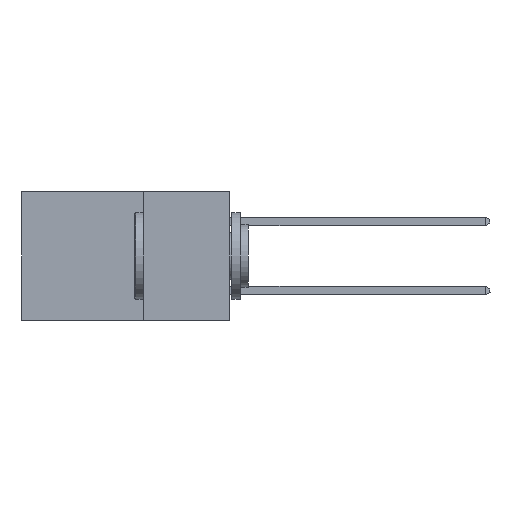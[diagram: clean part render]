
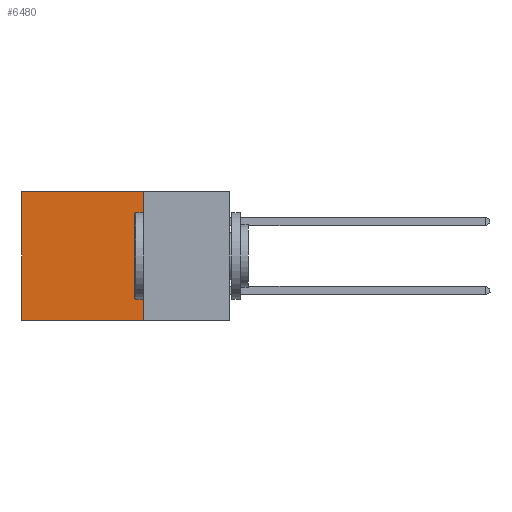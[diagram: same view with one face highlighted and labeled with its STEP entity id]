
A CAD part, left-side view. The second image highlights one B-rep face of the part: STEP entity #6480.
In plain terms, the highlighted planar face has unit normal (-1, 0, 0).
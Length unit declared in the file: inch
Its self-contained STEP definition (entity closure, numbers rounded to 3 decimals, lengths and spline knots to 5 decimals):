
#36 = FACE_OUTER_BOUND ( 'NONE', #13287, .T. ) ;
#1840 = LINE ( 'NONE', #17220, #14206 ) ;
#1922 = EDGE_CURVE ( 'NONE', #19029, #18520, #15356, .T. ) ;
#2025 = LINE ( 'NONE', #6024, #14391 ) ;
#2117 = CARTESIAN_POINT ( 'NONE',  ( 0.298, 0.25, -0.37 ) ) ;
#2572 = LINE ( 'NONE', #2117, #6442 ) ;
#2620 = ORIENTED_EDGE ( 'NONE', *, *, #1922, .T. ) ;
#6024 = CARTESIAN_POINT ( 'NONE',  ( 0.298, 0.25, 0. ) ) ;
#6319 = ORIENTED_EDGE ( 'NONE', *, *, #9165, .T. ) ;
#6348 = CARTESIAN_POINT ( 'NONE',  ( 0.298, 0.6, -0.37 ) ) ;
#6442 = VECTOR ( 'NONE', #8602, 39.37008 ) ;
#6480 = ADVANCED_FACE ( 'NONE', ( #36 ), #11713, .F. ) ;
#6762 = ORIENTED_EDGE ( 'NONE', *, *, #7657, .F. ) ;
#7228 = AXIS2_PLACEMENT_3D ( 'NONE', #13256, #11119, #13993 ) ;
#7657 = EDGE_CURVE ( 'NONE', #18199, #17182, #1840, .T. ) ;
#7661 = DIRECTION ( 'NONE',  ( 0., 1., 0. ) ) ;
#8280 = EDGE_CURVE ( 'NONE', #17182, #18520, #2572, .T. ) ;
#8602 = DIRECTION ( 'NONE',  ( 0., 1., 0. ) ) ;
#8672 = CARTESIAN_POINT ( 'NONE',  ( 0.298, 0.25, 0. ) ) ;
#9165 = EDGE_CURVE ( 'NONE', #18199, #19029, #2025, .T. ) ;
#9469 = CARTESIAN_POINT ( 'NONE',  ( 0.298, 0.6, 0. ) ) ;
#9495 = CARTESIAN_POINT ( 'NONE',  ( 0.298, 0.6, 0. ) ) ;
#9595 = CARTESIAN_POINT ( 'NONE',  ( 0.298, 0.25, -0.37 ) ) ;
#11119 = DIRECTION ( 'NONE',  ( 1., 0., 0. ) ) ;
#11713 = PLANE ( 'NONE',  #7228 ) ;
#13256 = CARTESIAN_POINT ( 'NONE',  ( 0.298, 0.25, 0. ) ) ;
#13287 = EDGE_LOOP ( 'NONE', ( #2620, #17744, #6762, #6319 ) ) ;
#13993 = DIRECTION ( 'NONE',  ( 0., 0., -1. ) ) ;
#14206 = VECTOR ( 'NONE', #16936, 39.37008 ) ;
#14391 = VECTOR ( 'NONE', #7661, 39.37008 ) ;
#15356 = LINE ( 'NONE', #9495, #19578 ) ;
#16936 = DIRECTION ( 'NONE',  ( 0., 0., -1. ) ) ;
#17182 = VERTEX_POINT ( 'NONE', #9595 ) ;
#17220 = CARTESIAN_POINT ( 'NONE',  ( 0.298, 0.25, 0. ) ) ;
#17423 = DIRECTION ( 'NONE',  ( 0., 0., -1. ) ) ;
#17744 = ORIENTED_EDGE ( 'NONE', *, *, #8280, .F. ) ;
#18199 = VERTEX_POINT ( 'NONE', #8672 ) ;
#18520 = VERTEX_POINT ( 'NONE', #6348 ) ;
#19029 = VERTEX_POINT ( 'NONE', #9469 ) ;
#19578 = VECTOR ( 'NONE', #17423, 39.37008 ) ;
